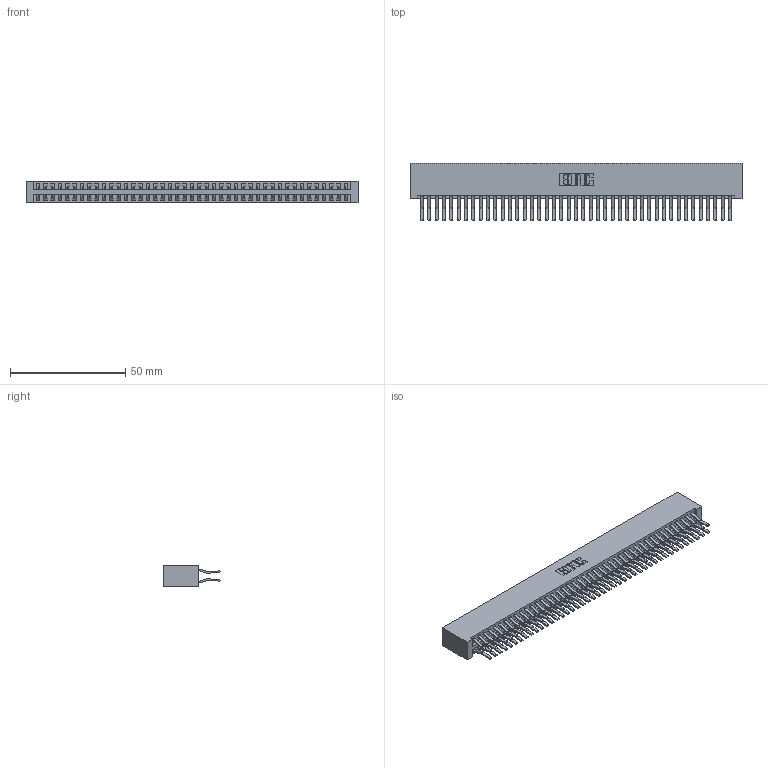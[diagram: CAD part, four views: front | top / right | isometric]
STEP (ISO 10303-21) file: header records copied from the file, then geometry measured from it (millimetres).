
FILE_DESCRIPTION (( 'STEP AP203' ), '1' );
FILE_NAME ('396-086-560-201.STEP', '2018-09-10T04:45:27', ( '' ), ( '' ), 'SwSTEP 2.0', 'SolidWorks 2016', '' );
FILE_SCHEMA (( 'CONFIG_CONTROL_DESIGN' ));
Length unit declared in the file: inch
Products named in the file (3): 346 Part_No Mounting Lugs; 345-292-001_560 Tail; 396-086-560-201
Assembly tree (87 placements, depth 2):
  396-086-560-201
    346 Part_No Mounting Lugs
    345-292-001_560 Tail  x86
Bounding box: 143.76 x 24.78 x 9.4 mm (x, y, z)
Volume: 15163.5 mm3; surface area: 22526.1 mm2
Topology: 87 solids, 87 shells, 4758 faces, 14151 edges, 9318 vertices
Faces by surface type: plane 3082, cylinder 1676
Entity records: 27739 total; most frequent: CARTESIAN_POINT 4568, ORIENTED_EDGE 4502, DIRECTION 4075, EDGE_CURVE 2251, VECTOR 1951, LINE 1951, VERTEX_POINT 1498, AXIS2_PLACEMENT_3D 1062
